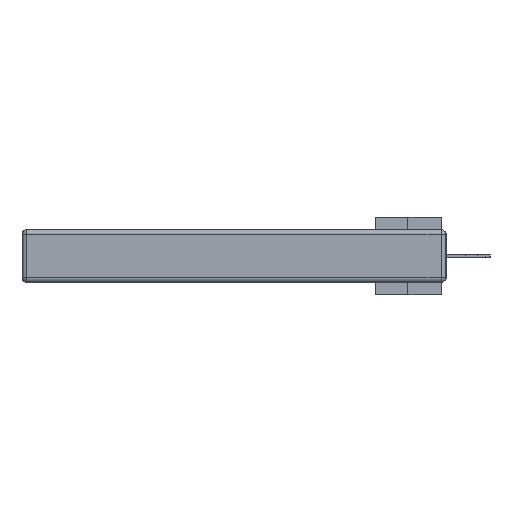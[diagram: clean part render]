
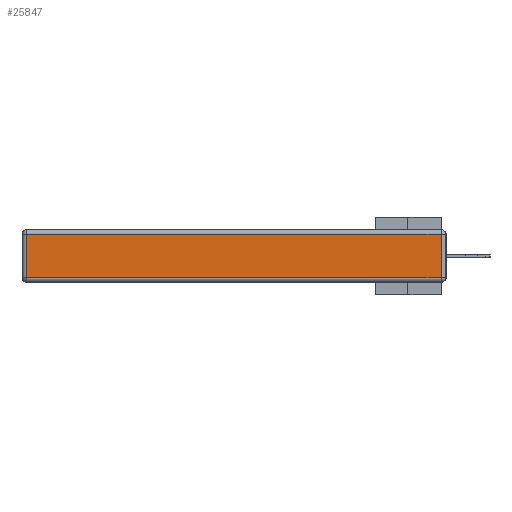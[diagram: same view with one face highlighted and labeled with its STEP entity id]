
A CAD part, left-side view. The second image highlights one B-rep face of the part: STEP entity #25847.
In plain terms, the highlighted planar face has unit normal (-1, 0, 0).
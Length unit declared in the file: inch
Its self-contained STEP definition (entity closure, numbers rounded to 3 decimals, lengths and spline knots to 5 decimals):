
#502 = VERTEX_POINT ( 'NONE', #24083 ) ;
#542 = CARTESIAN_POINT ( 'NONE',  ( 0., 2.75, -0.03 ) ) ;
#2925 = ORIENTED_EDGE ( 'NONE', *, *, #22683, .T. ) ;
#3640 = VECTOR ( 'NONE', #19262, 39.37008 ) ;
#4065 = CARTESIAN_POINT ( 'NONE',  ( 0., 0., -0.313 ) ) ;
#4246 = ORIENTED_EDGE ( 'NONE', *, *, #14161, .T. ) ;
#4598 = DIRECTION ( 'NONE',  ( 0., -1., 0. ) ) ;
#5872 = VECTOR ( 'NONE', #31525, 39.37008 ) ;
#6017 = DIRECTION ( 'NONE',  ( -1., 0., 0. ) ) ;
#8185 = LINE ( 'NONE', #36047, #3640 ) ;
#8496 = LINE ( 'NONE', #542, #5872 ) ;
#9154 = CARTESIAN_POINT ( 'NONE',  ( 0., 0., -0.343 ) ) ;
#9930 = AXIS2_PLACEMENT_3D ( 'NONE', #9154, #6017, #29262 ) ;
#10438 = VECTOR ( 'NONE', #4598, 39.37008 ) ;
#12690 = VERTEX_POINT ( 'NONE', #30537 ) ;
#14161 = EDGE_CURVE ( 'NONE', #16177, #34988, #15413, .T. ) ;
#15413 = LINE ( 'NONE', #34793, #21053 ) ;
#16177 = VERTEX_POINT ( 'NONE', #30855 ) ;
#17102 = CARTESIAN_POINT ( 'NONE',  ( 0., 0.03, -0.03 ) ) ;
#17105 = ORIENTED_EDGE ( 'NONE', *, *, #17820, .T. ) ;
#17820 = EDGE_CURVE ( 'NONE', #34988, #12690, #8496, .T. ) ;
#19262 = DIRECTION ( 'NONE',  ( 0., 0., -1. ) ) ;
#21053 = VECTOR ( 'NONE', #32396, 39.37008 ) ;
#22683 = EDGE_CURVE ( 'NONE', #502, #16177, #32640, .T. ) ;
#24083 = CARTESIAN_POINT ( 'NONE',  ( 0., 2.72, -0.313 ) ) ;
#25847 = ADVANCED_FACE ( 'NONE', ( #29069 ), #32026, .T. ) ;
#27957 = ORIENTED_EDGE ( 'NONE', *, *, #33008, .T. ) ;
#29069 = FACE_OUTER_BOUND ( 'NONE', #35279, .T. ) ;
#29262 = DIRECTION ( 'NONE',  ( 0., 0., 1. ) ) ;
#30537 = CARTESIAN_POINT ( 'NONE',  ( 0., 2.72, -0.03 ) ) ;
#30855 = CARTESIAN_POINT ( 'NONE',  ( 0., 0.03, -0.313 ) ) ;
#31525 = DIRECTION ( 'NONE',  ( 0., 1., 0. ) ) ;
#32026 = PLANE ( 'NONE',  #9930 ) ;
#32396 = DIRECTION ( 'NONE',  ( 0., 0., 1. ) ) ;
#32640 = LINE ( 'NONE', #4065, #10438 ) ;
#33008 = EDGE_CURVE ( 'NONE', #12690, #502, #8185, .T. ) ;
#34793 = CARTESIAN_POINT ( 'NONE',  ( 0., 0.03, -0.343 ) ) ;
#34988 = VERTEX_POINT ( 'NONE', #17102 ) ;
#35279 = EDGE_LOOP ( 'NONE', ( #2925, #4246, #17105, #27957 ) ) ;
#36047 = CARTESIAN_POINT ( 'NONE',  ( 0., 2.72, -0.343 ) ) ;
